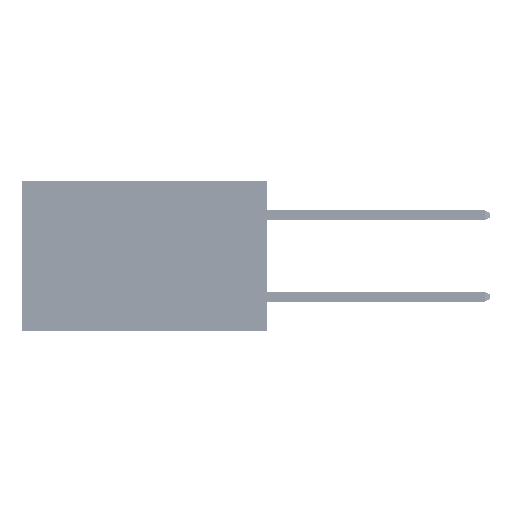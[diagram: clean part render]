
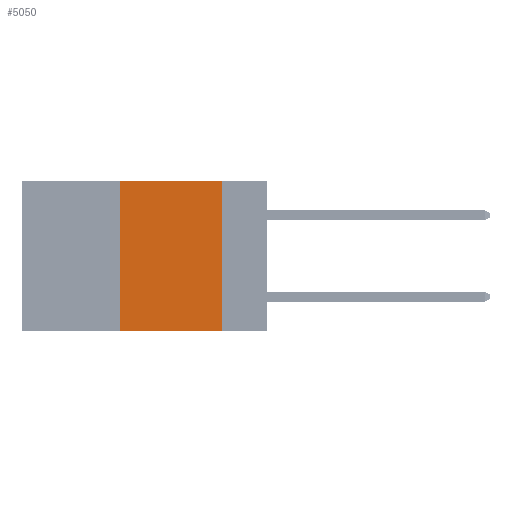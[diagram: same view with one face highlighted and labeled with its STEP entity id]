
A CAD part, left-side view. The second image highlights one B-rep face of the part: STEP entity #5050.
In plain terms, the highlighted planar face has unit normal (-1, 0, 0).
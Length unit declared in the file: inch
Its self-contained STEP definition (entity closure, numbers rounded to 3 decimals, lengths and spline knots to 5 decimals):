
#621 = VECTOR ( 'NONE', #34768, 39.37008 ) ;
#2486 = ORIENTED_EDGE ( 'NONE', *, *, #7927, .F. ) ;
#5050 = ADVANCED_FACE ( 'NONE', ( #6832 ), #17822, .F. ) ;
#6299 = LINE ( 'NONE', #45961, #621 ) ;
#6832 = FACE_OUTER_BOUND ( 'NONE', #29598, .T. ) ;
#6951 = EDGE_CURVE ( 'NONE', #39627, #38986, #14892, .T. ) ;
#7927 = EDGE_CURVE ( 'NONE', #19125, #39627, #6299, .T. ) ;
#9676 = DIRECTION ( 'NONE',  ( 0., -1., 0. ) ) ;
#10260 = CARTESIAN_POINT ( 'NONE',  ( 0., 0.36, 0. ) ) ;
#11261 = AXIS2_PLACEMENT_3D ( 'NONE', #46036, #32425, #38651 ) ;
#12938 = DIRECTION ( 'NONE',  ( 0., 0., 1. ) ) ;
#14892 = LINE ( 'NONE', #32609, #18104 ) ;
#16839 = CARTESIAN_POINT ( 'NONE',  ( 0., 0.6, -0.37 ) ) ;
#17822 = PLANE ( 'NONE',  #11261 ) ;
#18104 = VECTOR ( 'NONE', #21828, 39.37008 ) ;
#18754 = EDGE_CURVE ( 'NONE', #26203, #38986, #42873, .T. ) ;
#19125 = VERTEX_POINT ( 'NONE', #10260 ) ;
#20032 = VECTOR ( 'NONE', #9676, 39.37008 ) ;
#20327 = ORIENTED_EDGE ( 'NONE', *, *, #6951, .F. ) ;
#21828 = DIRECTION ( 'NONE',  ( 0., 0., -1. ) ) ;
#23679 = LINE ( 'NONE', #30158, #45133 ) ;
#25163 = ORIENTED_EDGE ( 'NONE', *, *, #41105, .F. ) ;
#25844 = CARTESIAN_POINT ( 'NONE',  ( 0., 0.11, 0. ) ) ;
#26203 = VERTEX_POINT ( 'NONE', #39387 ) ;
#29598 = EDGE_LOOP ( 'NONE', ( #20327, #2486, #25163, #37775 ) ) ;
#30158 = CARTESIAN_POINT ( 'NONE',  ( 0., 0.36, 0. ) ) ;
#30723 = CARTESIAN_POINT ( 'NONE',  ( 0., 0.11, -0.37 ) ) ;
#32425 = DIRECTION ( 'NONE',  ( 1., 0., 0. ) ) ;
#32609 = CARTESIAN_POINT ( 'NONE',  ( 0., 0.11, 0. ) ) ;
#34768 = DIRECTION ( 'NONE',  ( 0., -1., 0. ) ) ;
#37775 = ORIENTED_EDGE ( 'NONE', *, *, #18754, .T. ) ;
#38651 = DIRECTION ( 'NONE',  ( 0., 0., -1. ) ) ;
#38986 = VERTEX_POINT ( 'NONE', #30723 ) ;
#39387 = CARTESIAN_POINT ( 'NONE',  ( 0., 0.36, -0.37 ) ) ;
#39627 = VERTEX_POINT ( 'NONE', #25844 ) ;
#41105 = EDGE_CURVE ( 'NONE', #26203, #19125, #23679, .T. ) ;
#42873 = LINE ( 'NONE', #16839, #20032 ) ;
#45133 = VECTOR ( 'NONE', #12938, 39.37008 ) ;
#45961 = CARTESIAN_POINT ( 'NONE',  ( 0., 0.6, 0. ) ) ;
#46036 = CARTESIAN_POINT ( 'NONE',  ( 0., 0.6, 0. ) ) ;
